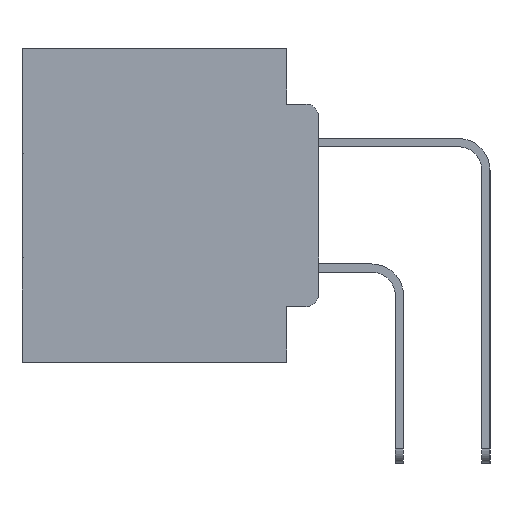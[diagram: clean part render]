
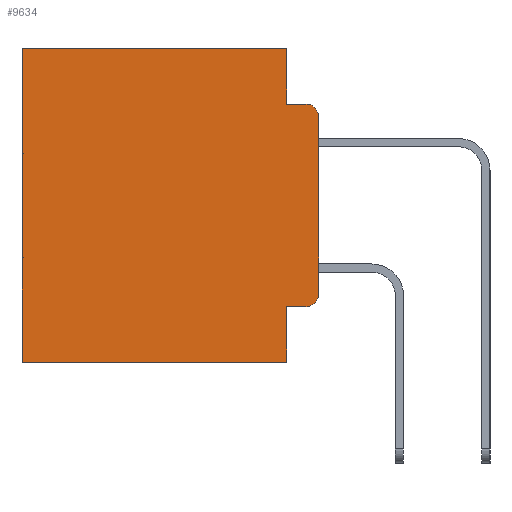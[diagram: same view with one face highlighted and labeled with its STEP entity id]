
A CAD part, left-side view. The second image highlights one B-rep face of the part: STEP entity #9634.
In plain terms, the highlighted planar face has unit normal (-1, 0, 0).
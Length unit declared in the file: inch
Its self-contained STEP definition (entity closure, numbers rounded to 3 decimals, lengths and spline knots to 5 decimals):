
#443 = CARTESIAN_POINT ( 'NONE',  ( 0.298, 0., -0.3915 ) ) ;
#502 = ORIENTED_EDGE ( 'NONE', *, *, #26127, .F. ) ;
#683 = CARTESIAN_POINT ( 'NONE',  ( 0.298, 0.051, 0. ) ) ;
#724 = CARTESIAN_POINT ( 'NONE',  ( 0.298, 0.051, -0.0885 ) ) ;
#1097 = LINE ( 'NONE', #4221, #31528 ) ;
#1633 = CARTESIAN_POINT ( 'NONE',  ( 0.298, 0., -0.1085 ) ) ;
#1739 = ORIENTED_EDGE ( 'NONE', *, *, #14689, .T. ) ;
#2297 = LINE ( 'NONE', #8215, #8192 ) ;
#2545 = ORIENTED_EDGE ( 'NONE', *, *, #15705, .T. ) ;
#2945 = VERTEX_POINT ( 'NONE', #15567 ) ;
#3460 = EDGE_CURVE ( 'NONE', #16143, #25662, #4386, .T. ) ;
#3879 = LINE ( 'NONE', #5443, #22744 ) ;
#3921 = VERTEX_POINT ( 'NONE', #31818 ) ;
#4057 = VECTOR ( 'NONE', #24818, 39.37008 ) ;
#4221 = CARTESIAN_POINT ( 'NONE',  ( 0.298, 0.051, 0. ) ) ;
#4260 = CARTESIAN_POINT ( 'NONE',  ( 0.298, 0.051, -0.0885 ) ) ;
#4386 = LINE ( 'NONE', #22353, #4057 ) ;
#4874 = ORIENTED_EDGE ( 'NONE', *, *, #27741, .T. ) ;
#5201 = DIRECTION ( 'NONE',  ( 0., 1., 0. ) ) ;
#5221 = DIRECTION ( 'NONE',  ( -1., 0., 0. ) ) ;
#5443 = CARTESIAN_POINT ( 'NONE',  ( 0.298, 0., 0. ) ) ;
#6193 = EDGE_CURVE ( 'NONE', #23260, #6211, #3879, .T. ) ;
#6211 = VERTEX_POINT ( 'NONE', #443 ) ;
#6249 = EDGE_CURVE ( 'NONE', #25063, #3921, #2297, .T. ) ;
#6329 = CARTESIAN_POINT ( 'NONE',  ( 0.298, 0., 0. ) ) ;
#6449 = PLANE ( 'NONE',  #26389 ) ;
#7043 = CARTESIAN_POINT ( 'NONE',  ( 0.298, 0.02, -0.3915 ) ) ;
#7453 = EDGE_CURVE ( 'NONE', #29287, #11146, #20042, .T. ) ;
#7996 = DIRECTION ( 'NONE',  ( 0., 0., -1. ) ) ;
#8089 = FACE_OUTER_BOUND ( 'NONE', #17628, .T. ) ;
#8192 = VECTOR ( 'NONE', #22872, 39.37008 ) ;
#8215 = CARTESIAN_POINT ( 'NONE',  ( 0.298, 0., -0.5 ) ) ;
#8982 = DIRECTION ( 'NONE',  ( 0., 0., -1. ) ) ;
#9078 = DIRECTION ( 'NONE',  ( 0., 0., -1. ) ) ;
#9594 = DIRECTION ( 'NONE',  ( 0., 0., -1. ) ) ;
#9634 = ADVANCED_FACE ( 'NONE', ( #8089 ), #6449, .F. ) ;
#9968 = AXIS2_PLACEMENT_3D ( 'NONE', #19963, #5221, #22431 ) ;
#10581 = VECTOR ( 'NONE', #27920, 39.37008 ) ;
#10887 = CARTESIAN_POINT ( 'NONE',  ( 0.298, 0.473, 0. ) ) ;
#11146 = VERTEX_POINT ( 'NONE', #21798 ) ;
#11996 = ORIENTED_EDGE ( 'NONE', *, *, #25514, .F. ) ;
#12878 = VECTOR ( 'NONE', #30310, 39.37008 ) ;
#14639 = ORIENTED_EDGE ( 'NONE', *, *, #7453, .F. ) ;
#14689 = EDGE_CURVE ( 'NONE', #23260, #11146, #17734, .T. ) ;
#15567 = CARTESIAN_POINT ( 'NONE',  ( 0.298, 0.051, 0. ) ) ;
#15705 = EDGE_CURVE ( 'NONE', #25662, #6211, #21113, .T. ) ;
#16143 = VERTEX_POINT ( 'NONE', #16177 ) ;
#16177 = CARTESIAN_POINT ( 'NONE',  ( 0.298, 0.051, -0.4115 ) ) ;
#16537 = VECTOR ( 'NONE', #5201, 39.37008 ) ;
#17013 = LINE ( 'NONE', #683, #10581 ) ;
#17628 = EDGE_LOOP ( 'NONE', ( #31012, #1739, #14639, #502, #4874, #19577, #24503, #11996, #22980, #2545 ) ) ;
#17734 = CIRCLE ( 'NONE', #9968, 0.02 ) ;
#18487 = VERTEX_POINT ( 'NONE', #10887 ) ;
#19577 = ORIENTED_EDGE ( 'NONE', *, *, #23886, .T. ) ;
#19963 = CARTESIAN_POINT ( 'NONE',  ( 0.298, 0.02, -0.1085 ) ) ;
#20042 = LINE ( 'NONE', #724, #12878 ) ;
#20713 = LINE ( 'NONE', #23716, #27233 ) ;
#21113 = CIRCLE ( 'NONE', #27797, 0.02 ) ;
#21426 = DIRECTION ( 'NONE',  ( 0., 0., -1. ) ) ;
#21798 = CARTESIAN_POINT ( 'NONE',  ( 0.298, 0.02, -0.0885 ) ) ;
#22353 = CARTESIAN_POINT ( 'NONE',  ( 0.298, 0.051, -0.4115 ) ) ;
#22408 = CARTESIAN_POINT ( 'NONE',  ( 0.298, 0., 0. ) ) ;
#22431 = DIRECTION ( 'NONE',  ( 0., 0., -1. ) ) ;
#22744 = VECTOR ( 'NONE', #7996, 39.37008 ) ;
#22872 = DIRECTION ( 'NONE',  ( 0., 1., 0. ) ) ;
#22980 = ORIENTED_EDGE ( 'NONE', *, *, #3460, .T. ) ;
#23260 = VERTEX_POINT ( 'NONE', #1633 ) ;
#23621 = CARTESIAN_POINT ( 'NONE',  ( 0.298, 0.02, -0.4115 ) ) ;
#23623 = DIRECTION ( 'NONE',  ( 1., 0., 0. ) ) ;
#23655 = CARTESIAN_POINT ( 'NONE',  ( 0.298, 0.051, -0.5 ) ) ;
#23716 = CARTESIAN_POINT ( 'NONE',  ( 0.298, 0.473, 0. ) ) ;
#23886 = EDGE_CURVE ( 'NONE', #18487, #3921, #20713, .T. ) ;
#24209 = DIRECTION ( 'NONE',  ( -1., 0., 0. ) ) ;
#24503 = ORIENTED_EDGE ( 'NONE', *, *, #6249, .F. ) ;
#24818 = DIRECTION ( 'NONE',  ( 0., -1., 0. ) ) ;
#25063 = VERTEX_POINT ( 'NONE', #23655 ) ;
#25514 = EDGE_CURVE ( 'NONE', #16143, #25063, #17013, .T. ) ;
#25662 = VERTEX_POINT ( 'NONE', #23621 ) ;
#26127 = EDGE_CURVE ( 'NONE', #2945, #29287, #1097, .T. ) ;
#26389 = AXIS2_PLACEMENT_3D ( 'NONE', #6329, #23623, #8982 ) ;
#27233 = VECTOR ( 'NONE', #9078, 39.37008 ) ;
#27741 = EDGE_CURVE ( 'NONE', #2945, #18487, #29560, .T. ) ;
#27797 = AXIS2_PLACEMENT_3D ( 'NONE', #7043, #24209, #9594 ) ;
#27920 = DIRECTION ( 'NONE',  ( 0., 0., -1. ) ) ;
#29287 = VERTEX_POINT ( 'NONE', #4260 ) ;
#29560 = LINE ( 'NONE', #22408, #16537 ) ;
#30310 = DIRECTION ( 'NONE',  ( 0., -1., 0. ) ) ;
#31012 = ORIENTED_EDGE ( 'NONE', *, *, #6193, .F. ) ;
#31528 = VECTOR ( 'NONE', #21426, 39.37008 ) ;
#31818 = CARTESIAN_POINT ( 'NONE',  ( 0.298, 0.473, -0.5 ) ) ;
